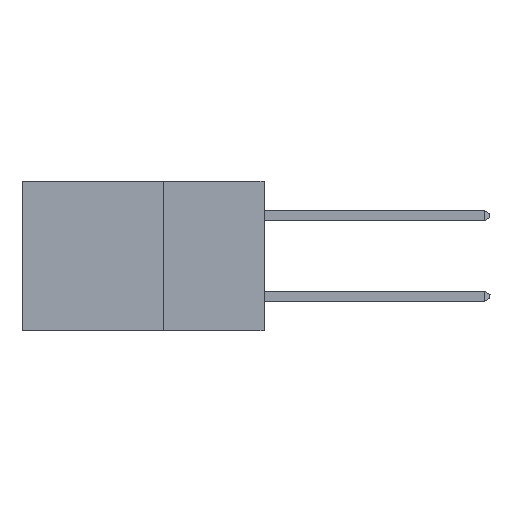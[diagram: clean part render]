
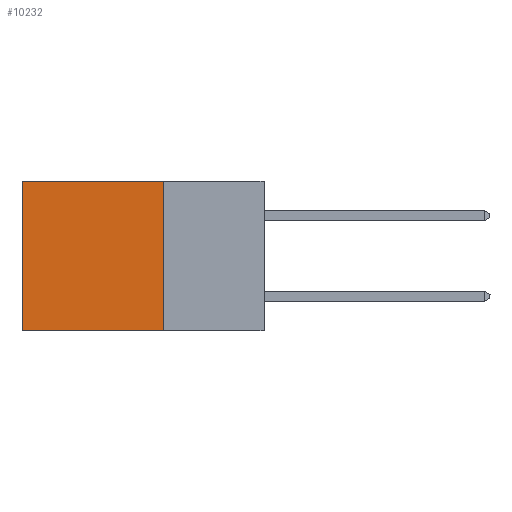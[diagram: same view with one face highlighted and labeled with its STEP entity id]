
A CAD part, left-side view. The second image highlights one B-rep face of the part: STEP entity #10232.
In plain terms, the highlighted planar face has unit normal (-1, 0, 0).
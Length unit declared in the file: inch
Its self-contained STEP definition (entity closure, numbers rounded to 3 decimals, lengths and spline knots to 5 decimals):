
#193 = VERTEX_POINT ( 'NONE', #3027 ) ;
#254 = VERTEX_POINT ( 'NONE', #496 ) ;
#458 = CARTESIAN_POINT ( 'NONE',  ( 0.298, 0.25, -0.37 ) ) ;
#496 = CARTESIAN_POINT ( 'NONE',  ( 0.298, 0.6, 0. ) ) ;
#513 = DIRECTION ( 'NONE',  ( 0., 1., 0. ) ) ;
#1053 = EDGE_CURVE ( 'NONE', #9891, #254, #15858, .T. ) ;
#1059 = ORIENTED_EDGE ( 'NONE', *, *, #1053, .T. ) ;
#2154 = CARTESIAN_POINT ( 'NONE',  ( 0.298, 0.25, 0. ) ) ;
#2289 = CARTESIAN_POINT ( 'NONE',  ( 0.298, 0.6, 0. ) ) ;
#2303 = ORIENTED_EDGE ( 'NONE', *, *, #5270, .F. ) ;
#2855 = CARTESIAN_POINT ( 'NONE',  ( 0.298, 0.25, 0. ) ) ;
#3027 = CARTESIAN_POINT ( 'NONE',  ( 0.298, 0.6, -0.37 ) ) ;
#3260 = LINE ( 'NONE', #458, #15890 ) ;
#4363 = LINE ( 'NONE', #2289, #9687 ) ;
#4537 = DIRECTION ( 'NONE',  ( 0., 0., -1. ) ) ;
#5270 = EDGE_CURVE ( 'NONE', #5810, #193, #3260, .T. ) ;
#5810 = VERTEX_POINT ( 'NONE', #10337 ) ;
#6258 = VECTOR ( 'NONE', #4537, 39.37008 ) ;
#6443 = PLANE ( 'NONE',  #8511 ) ;
#6904 = EDGE_LOOP ( 'NONE', ( #15383, #2303, #13629, #1059 ) ) ;
#8511 = AXIS2_PLACEMENT_3D ( 'NONE', #2855, #10389, #14084 ) ;
#8713 = VECTOR ( 'NONE', #513, 39.37008 ) ;
#8853 = EDGE_CURVE ( 'NONE', #254, #193, #4363, .T. ) ;
#9687 = VECTOR ( 'NONE', #13746, 39.37008 ) ;
#9891 = VERTEX_POINT ( 'NONE', #2154 ) ;
#10232 = ADVANCED_FACE ( 'NONE', ( #11410 ), #6443, .F. ) ;
#10337 = CARTESIAN_POINT ( 'NONE',  ( 0.298, 0.25, -0.37 ) ) ;
#10388 = LINE ( 'NONE', #14676, #6258 ) ;
#10389 = DIRECTION ( 'NONE',  ( 1., 0., 0. ) ) ;
#10635 = CARTESIAN_POINT ( 'NONE',  ( 0.298, 0.25, 0. ) ) ;
#11410 = FACE_OUTER_BOUND ( 'NONE', #6904, .T. ) ;
#11737 = DIRECTION ( 'NONE',  ( 0., 1., 0. ) ) ;
#13629 = ORIENTED_EDGE ( 'NONE', *, *, #15833, .F. ) ;
#13746 = DIRECTION ( 'NONE',  ( 0., 0., -1. ) ) ;
#14084 = DIRECTION ( 'NONE',  ( 0., 0., -1. ) ) ;
#14676 = CARTESIAN_POINT ( 'NONE',  ( 0.298, 0.25, 0. ) ) ;
#15383 = ORIENTED_EDGE ( 'NONE', *, *, #8853, .T. ) ;
#15833 = EDGE_CURVE ( 'NONE', #9891, #5810, #10388, .T. ) ;
#15858 = LINE ( 'NONE', #10635, #8713 ) ;
#15890 = VECTOR ( 'NONE', #11737, 39.37008 ) ;
